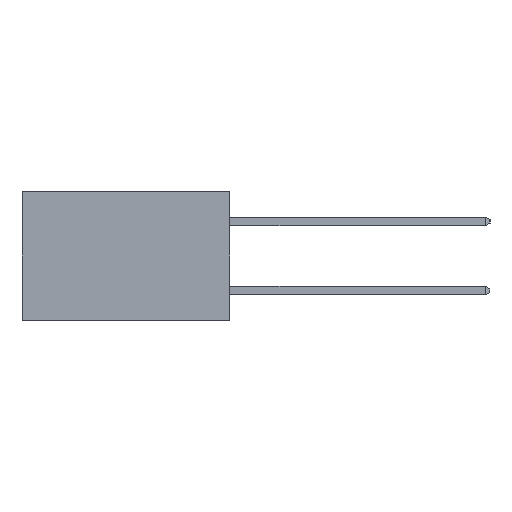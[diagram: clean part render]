
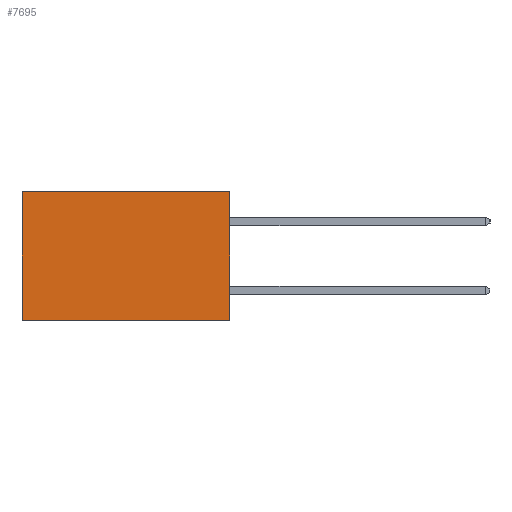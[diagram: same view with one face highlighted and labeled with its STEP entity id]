
A CAD part, left-side view. The second image highlights one B-rep face of the part: STEP entity #7695.
In plain terms, the highlighted planar face has unit normal (-1, 0, 0).
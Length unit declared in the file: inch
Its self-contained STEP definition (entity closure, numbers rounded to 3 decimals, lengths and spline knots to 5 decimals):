
#137 = LINE ( 'NONE', #17252, #9294 ) ;
#675 = VECTOR ( 'NONE', #13310, 39.37008 ) ;
#1195 = DIRECTION ( 'NONE',  ( 1., 0., 0. ) ) ;
#2177 = VERTEX_POINT ( 'NONE', #19933 ) ;
#2299 = ORIENTED_EDGE ( 'NONE', *, *, #4237, .T. ) ;
#2312 = EDGE_CURVE ( 'NONE', #17947, #2177, #13894, .T. ) ;
#4237 = EDGE_CURVE ( 'NONE', #17947, #16244, #137, .T. ) ;
#4465 = VECTOR ( 'NONE', #20553, 39.37008 ) ;
#4522 = VECTOR ( 'NONE', #12317, 39.37008 ) ;
#4608 = CARTESIAN_POINT ( 'NONE',  ( 0.298, 0., 0. ) ) ;
#4735 = ORIENTED_EDGE ( 'NONE', *, *, #5113, .T. ) ;
#5113 = EDGE_CURVE ( 'NONE', #16244, #15334, #14893, .T. ) ;
#5293 = CARTESIAN_POINT ( 'NONE',  ( 0.298, 0.6, -0.37 ) ) ;
#7695 = ADVANCED_FACE ( 'NONE', ( #12007 ), #10024, .F. ) ;
#8719 = LINE ( 'NONE', #20525, #4465 ) ;
#9294 = VECTOR ( 'NONE', #17146, 39.37008 ) ;
#9368 = EDGE_CURVE ( 'NONE', #2177, #15334, #8719, .T. ) ;
#10024 = PLANE ( 'NONE',  #17350 ) ;
#12007 = FACE_OUTER_BOUND ( 'NONE', #14140, .T. ) ;
#12035 = DIRECTION ( 'NONE',  ( 0., 0., -1. ) ) ;
#12317 = DIRECTION ( 'NONE',  ( 0., 0., -1. ) ) ;
#13310 = DIRECTION ( 'NONE',  ( 0., 0., -1. ) ) ;
#13738 = CARTESIAN_POINT ( 'NONE',  ( 0.298, 0.6, 0. ) ) ;
#13894 = LINE ( 'NONE', #20819, #4522 ) ;
#14140 = EDGE_LOOP ( 'NONE', ( #4735, #17245, #19707, #2299 ) ) ;
#14893 = LINE ( 'NONE', #13738, #675 ) ;
#15334 = VERTEX_POINT ( 'NONE', #5293 ) ;
#16244 = VERTEX_POINT ( 'NONE', #20932 ) ;
#17146 = DIRECTION ( 'NONE',  ( 0., 1., 0. ) ) ;
#17245 = ORIENTED_EDGE ( 'NONE', *, *, #9368, .F. ) ;
#17252 = CARTESIAN_POINT ( 'NONE',  ( 0.298, 0., 0. ) ) ;
#17350 = AXIS2_PLACEMENT_3D ( 'NONE', #20799, #1195, #12035 ) ;
#17947 = VERTEX_POINT ( 'NONE', #4608 ) ;
#19707 = ORIENTED_EDGE ( 'NONE', *, *, #2312, .F. ) ;
#19933 = CARTESIAN_POINT ( 'NONE',  ( 0.298, 0., -0.37 ) ) ;
#20525 = CARTESIAN_POINT ( 'NONE',  ( 0.298, 0., -0.37 ) ) ;
#20553 = DIRECTION ( 'NONE',  ( 0., 1., 0. ) ) ;
#20799 = CARTESIAN_POINT ( 'NONE',  ( 0.298, 0., 0. ) ) ;
#20819 = CARTESIAN_POINT ( 'NONE',  ( 0.298, 0., 0. ) ) ;
#20932 = CARTESIAN_POINT ( 'NONE',  ( 0.298, 0.6, 0. ) ) ;
